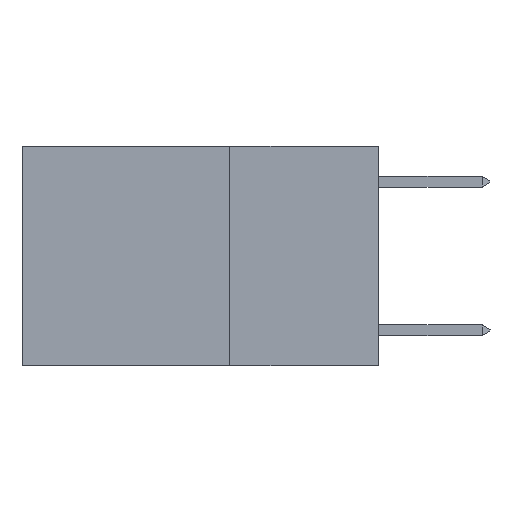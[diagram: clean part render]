
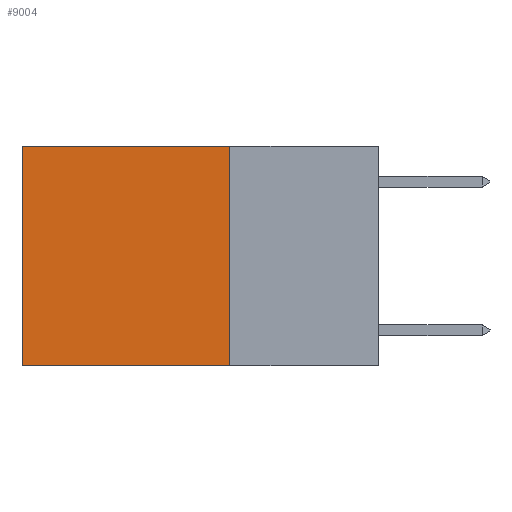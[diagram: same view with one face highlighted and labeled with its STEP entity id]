
A CAD part, left-side view. The second image highlights one B-rep face of the part: STEP entity #9004.
In plain terms, the highlighted planar face has unit normal (-1, 0, 0).
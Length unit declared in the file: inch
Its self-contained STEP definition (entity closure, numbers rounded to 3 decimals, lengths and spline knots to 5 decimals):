
#186 = CARTESIAN_POINT ( 'NONE',  ( 0.2625, 0.25, 0. ) ) ;
#659 = LINE ( 'NONE', #2317, #3647 ) ;
#881 = ORIENTED_EDGE ( 'NONE', *, *, #9098, .F. ) ;
#1353 = CARTESIAN_POINT ( 'NONE',  ( 0.2625, 0.6, 0. ) ) ;
#1645 = EDGE_CURVE ( 'NONE', #7994, #9274, #6569, .T. ) ;
#1895 = DIRECTION ( 'NONE',  ( 0., 1., 0. ) ) ;
#2317 = CARTESIAN_POINT ( 'NONE',  ( 0.2625, 0.25, -0.37 ) ) ;
#2860 = PLANE ( 'NONE',  #8271 ) ;
#3171 = CARTESIAN_POINT ( 'NONE',  ( 0.2625, 0.25, 0. ) ) ;
#3647 = VECTOR ( 'NONE', #11695, 39.37008 ) ;
#3669 = CARTESIAN_POINT ( 'NONE',  ( 0.2625, 0.6, 0. ) ) ;
#4251 = CARTESIAN_POINT ( 'NONE',  ( 0.2625, 0.25, 0. ) ) ;
#5233 = FACE_OUTER_BOUND ( 'NONE', #10301, .T. ) ;
#5452 = DIRECTION ( 'NONE',  ( 0., 0., -1. ) ) ;
#5578 = EDGE_CURVE ( 'NONE', #10072, #12243, #659, .T. ) ;
#5667 = EDGE_CURVE ( 'NONE', #9274, #12243, #12191, .T. ) ;
#6103 = CARTESIAN_POINT ( 'NONE',  ( 0.2625, 0.25, -0.37 ) ) ;
#6448 = DIRECTION ( 'NONE',  ( 1., 0., 0. ) ) ;
#6569 = LINE ( 'NONE', #3171, #9319 ) ;
#6892 = LINE ( 'NONE', #4251, #12601 ) ;
#7994 = VERTEX_POINT ( 'NONE', #186 ) ;
#8271 = AXIS2_PLACEMENT_3D ( 'NONE', #13288, #6448, #14423 ) ;
#9004 = ADVANCED_FACE ( 'NONE', ( #5233 ), #2860, .F. ) ;
#9098 = EDGE_CURVE ( 'NONE', #7994, #10072, #6892, .T. ) ;
#9210 = VECTOR ( 'NONE', #15188, 39.37008 ) ;
#9274 = VERTEX_POINT ( 'NONE', #1353 ) ;
#9319 = VECTOR ( 'NONE', #1895, 39.37008 ) ;
#10022 = CARTESIAN_POINT ( 'NONE',  ( 0.2625, 0.6, -0.37 ) ) ;
#10072 = VERTEX_POINT ( 'NONE', #6103 ) ;
#10125 = ORIENTED_EDGE ( 'NONE', *, *, #5578, .F. ) ;
#10301 = EDGE_LOOP ( 'NONE', ( #12717, #10125, #881, #13448 ) ) ;
#11695 = DIRECTION ( 'NONE',  ( 0., 1., 0. ) ) ;
#12191 = LINE ( 'NONE', #3669, #9210 ) ;
#12243 = VERTEX_POINT ( 'NONE', #10022 ) ;
#12601 = VECTOR ( 'NONE', #5452, 39.37008 ) ;
#12717 = ORIENTED_EDGE ( 'NONE', *, *, #5667, .T. ) ;
#13288 = CARTESIAN_POINT ( 'NONE',  ( 0.2625, 0.25, 0. ) ) ;
#13448 = ORIENTED_EDGE ( 'NONE', *, *, #1645, .T. ) ;
#14423 = DIRECTION ( 'NONE',  ( 0., 0., -1. ) ) ;
#15188 = DIRECTION ( 'NONE',  ( 0., 0., -1. ) ) ;
